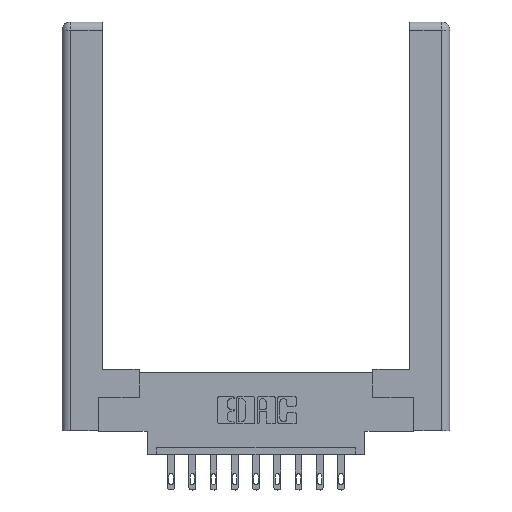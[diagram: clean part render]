
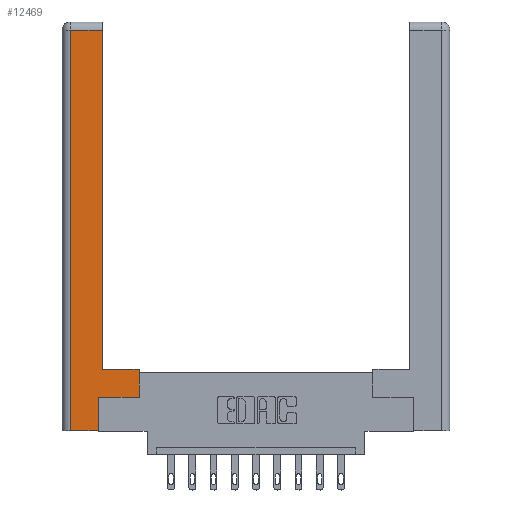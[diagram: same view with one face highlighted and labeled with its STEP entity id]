
A CAD part, top view. The second image highlights one B-rep face of the part: STEP entity #12469.
In plain terms, the highlighted planar face has unit normal (0, 0, 1).
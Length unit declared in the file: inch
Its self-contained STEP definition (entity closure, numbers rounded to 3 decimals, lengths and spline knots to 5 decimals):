
#299 = ORIENTED_EDGE ( 'NONE', *, *, #5805, .T. ) ;
#419 = EDGE_CURVE ( 'NONE', #9266, #2146, #922, .T. ) ;
#521 = VECTOR ( 'NONE', #13384, 39.37008 ) ;
#702 = VERTEX_POINT ( 'NONE', #4071 ) ;
#802 = ORIENTED_EDGE ( 'NONE', *, *, #3255, .T. ) ;
#879 = CARTESIAN_POINT ( 'NONE',  ( 0.295, 3., 0. ) ) ;
#922 = LINE ( 'NONE', #8614, #6042 ) ;
#981 = CARTESIAN_POINT ( 'NONE',  ( 0.0615, 2.94, 0. ) ) ;
#1450 = DIRECTION ( 'NONE',  ( -1., 0., 0. ) ) ;
#1509 = DIRECTION ( 'NONE',  ( 1., 0., 0. ) ) ;
#1610 = EDGE_CURVE ( 'NONE', #2146, #5025, #5342, .T. ) ;
#2146 = VERTEX_POINT ( 'NONE', #9305 ) ;
#2159 = CARTESIAN_POINT ( 'NONE',  ( 0.265, 0.245, 0. ) ) ;
#2246 = ORIENTED_EDGE ( 'NONE', *, *, #11097, .T. ) ;
#2578 = DIRECTION ( 'NONE',  ( 0., 1., 0. ) ) ;
#2647 = VECTOR ( 'NONE', #3336, 39.37008 ) ;
#2675 = ORIENTED_EDGE ( 'NONE', *, *, #9800, .T. ) ;
#2730 = ORIENTED_EDGE ( 'NONE', *, *, #3305, .T. ) ;
#3164 = VECTOR ( 'NONE', #10336, 39.37008 ) ;
#3205 = CARTESIAN_POINT ( 'NONE',  ( 0.265, 0.245, 0. ) ) ;
#3255 = EDGE_CURVE ( 'NONE', #8299, #9266, #6682, .T. ) ;
#3305 = EDGE_CURVE ( 'NONE', #5270, #8911, #5546, .T. ) ;
#3336 = DIRECTION ( 'NONE',  ( -1., 0., 0. ) ) ;
#3625 = ORIENTED_EDGE ( 'NONE', *, *, #1610, .T. ) ;
#3931 = CARTESIAN_POINT ( 'NONE',  ( 0., 0., 0. ) ) ;
#4071 = CARTESIAN_POINT ( 'NONE',  ( 0.295, 0.45, 0. ) ) ;
#5025 = VERTEX_POINT ( 'NONE', #13132 ) ;
#5228 = VECTOR ( 'NONE', #2578, 39.37008 ) ;
#5270 = VERTEX_POINT ( 'NONE', #10101 ) ;
#5342 = LINE ( 'NONE', #13499, #3164 ) ;
#5546 = LINE ( 'NONE', #6744, #5228 ) ;
#5595 = DIRECTION ( 'NONE',  ( 0., -1., 0. ) ) ;
#5725 = ORIENTED_EDGE ( 'NONE', *, *, #419, .T. ) ;
#5805 = EDGE_CURVE ( 'NONE', #8911, #702, #7457, .T. ) ;
#6042 = VECTOR ( 'NONE', #5595, 39.37008 ) ;
#6421 = DIRECTION ( 'NONE',  ( 0., 1., 0. ) ) ;
#6682 = LINE ( 'NONE', #7757, #11816 ) ;
#6744 = CARTESIAN_POINT ( 'NONE',  ( 0.565, 0.45, 0. ) ) ;
#7457 = LINE ( 'NONE', #12824, #2647 ) ;
#7714 = LINE ( 'NONE', #3205, #11020 ) ;
#7757 = CARTESIAN_POINT ( 'NONE',  ( 0.0615, 2.94, 0. ) ) ;
#8299 = VERTEX_POINT ( 'NONE', #9140 ) ;
#8404 = LINE ( 'NONE', #879, #521 ) ;
#8614 = CARTESIAN_POINT ( 'NONE',  ( 0.0615, 0., 0. ) ) ;
#8911 = VERTEX_POINT ( 'NONE', #13218 ) ;
#9140 = CARTESIAN_POINT ( 'NONE',  ( 0.295, 2.94, 0. ) ) ;
#9228 = PLANE ( 'NONE',  #12844 ) ;
#9266 = VERTEX_POINT ( 'NONE', #981 ) ;
#9305 = CARTESIAN_POINT ( 'NONE',  ( 0.0615, 0., 0. ) ) ;
#9800 = EDGE_CURVE ( 'NONE', #702, #8299, #8404, .T. ) ;
#9981 = VECTOR ( 'NONE', #1509, 39.37008 ) ;
#10101 = CARTESIAN_POINT ( 'NONE',  ( 0.565, 0.245, 0. ) ) ;
#10336 = DIRECTION ( 'NONE',  ( 1., 0., 0. ) ) ;
#10513 = VERTEX_POINT ( 'NONE', #2159 ) ;
#10905 = CARTESIAN_POINT ( 'NONE',  ( 0.565, 0.245, 0. ) ) ;
#11020 = VECTOR ( 'NONE', #6421, 39.37008 ) ;
#11097 = EDGE_CURVE ( 'NONE', #5025, #10513, #7714, .T. ) ;
#11410 = DIRECTION ( 'NONE',  ( -1., 0., 0. ) ) ;
#11624 = LINE ( 'NONE', #10905, #9981 ) ;
#11716 = ORIENTED_EDGE ( 'NONE', *, *, #13365, .T. ) ;
#11816 = VECTOR ( 'NONE', #1450, 39.37008 ) ;
#12379 = DIRECTION ( 'NONE',  ( 0., 0., -1. ) ) ;
#12469 = ADVANCED_FACE ( 'NONE', ( #13320 ), #9228, .F. ) ;
#12824 = CARTESIAN_POINT ( 'NONE',  ( 0.295, 0.45, 0. ) ) ;
#12844 = AXIS2_PLACEMENT_3D ( 'NONE', #3931, #12379, #11410 ) ;
#12928 = EDGE_LOOP ( 'NONE', ( #2675, #802, #5725, #3625, #2246, #11716, #2730, #299 ) ) ;
#13132 = CARTESIAN_POINT ( 'NONE',  ( 0.265, 0., 0. ) ) ;
#13218 = CARTESIAN_POINT ( 'NONE',  ( 0.565, 0.45, 0. ) ) ;
#13320 = FACE_OUTER_BOUND ( 'NONE', #12928, .T. ) ;
#13365 = EDGE_CURVE ( 'NONE', #10513, #5270, #11624, .T. ) ;
#13384 = DIRECTION ( 'NONE',  ( 0., 1., 0. ) ) ;
#13499 = CARTESIAN_POINT ( 'NONE',  ( 0.265, 0., 0. ) ) ;
